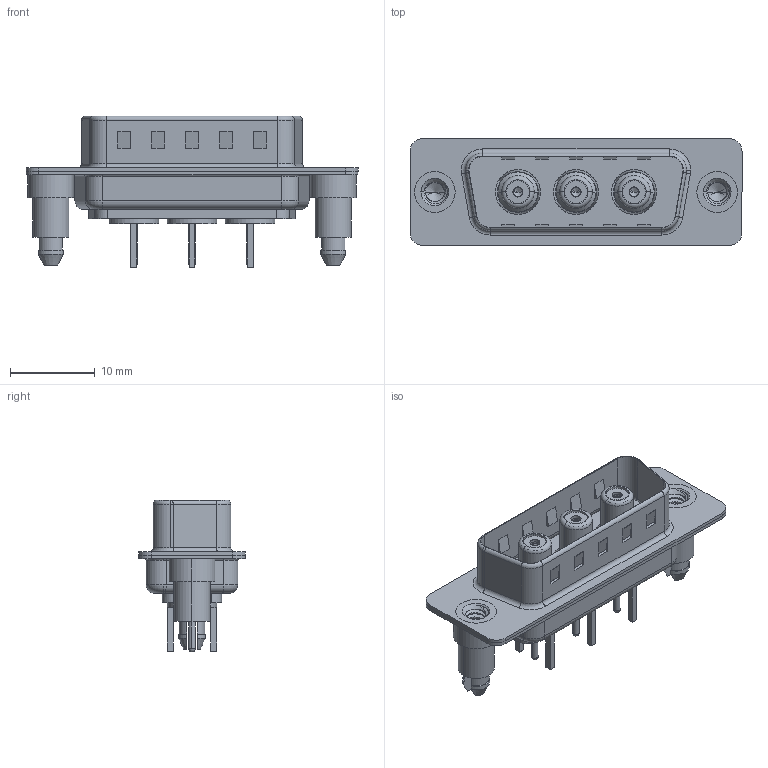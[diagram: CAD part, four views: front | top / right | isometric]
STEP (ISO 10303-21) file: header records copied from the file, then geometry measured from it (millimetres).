
FILE_DESCRIPTION (( 'STEP AP203' ), '1' );
FILE_NAME ('627-3W3-624-5T5.STEP', '2019-05-24T18:50:52', ( '' ), ( '' ), 'SwSTEP 2.0', 'SolidWorks 2016', '' );
FILE_SCHEMA (( 'CONFIG_CONTROL_DESIGN' ));
Length unit declared in the file: millimetre
Products named in the file (11): 627-3W3-624-5T5; 627Combo Shell Front_15 Contacts; 627Combo Threaded Boardlock_5; Co-Ax Jack_Straight PC Tail; Insulator Socket; Insulator Socket 2; Locking Collar; Socket_Str; 627Combo Housing_3W3; Co-Ax Jack Assy_S; 627Combo Shell Rear_15 Contacts
Assembly tree (13 placements, depth 3):
  627-3W3-624-5T5
    627Combo Housing_3W3
    627Combo Shell Rear_15 Contacts
    627Combo Shell Front_15 Contacts
    627Combo Threaded Boardlock_5  x2
    Co-Ax Jack Assy_S  x3
      Co-Ax Jack_Straight PC Tail
      Insulator Socket
      Insulator Socket 2
      Locking Collar
      Socket_Str
Bounding box: 39.15 x 12.6 x 17.9 mm (x, y, z)
Volume: 2041.2 mm3; surface area: 6253.5 mm2
Topology: 20 solids, 20 shells, 723 faces, 1736 edges, 1092 vertices
Faces by surface type: cylinder 306, plane 296, torus 62, cone 41, bspline 12, sphere 6
Entity records: 16310 total; most frequent: CARTESIAN_POINT 4136, DIRECTION 2380, ORIENTED_EDGE 2214, EDGE_CURVE 1107, AXIS2_PLACEMENT_3D 892, VERTEX_POINT 701, VECTOR 596, LINE 596
